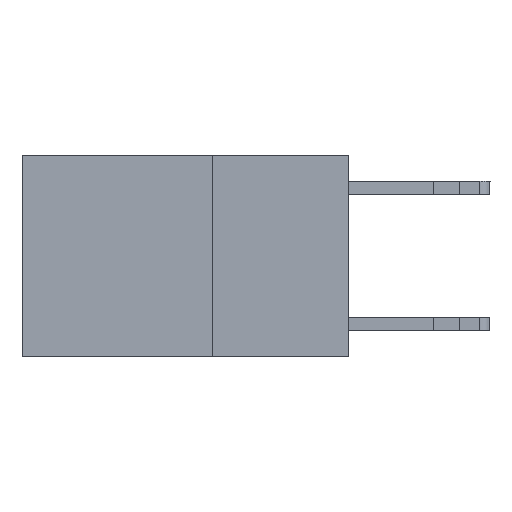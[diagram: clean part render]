
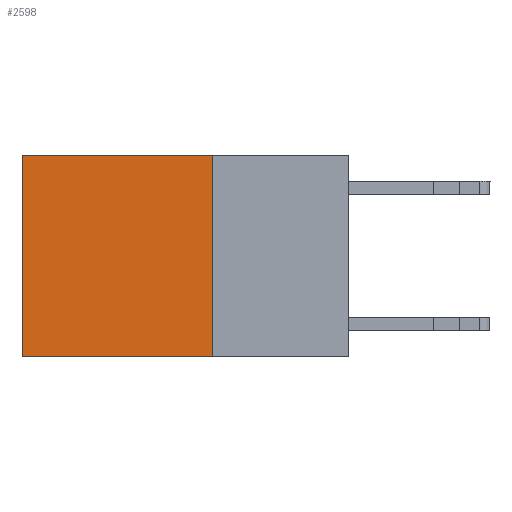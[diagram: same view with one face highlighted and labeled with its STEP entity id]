
A CAD part, left-side view. The second image highlights one B-rep face of the part: STEP entity #2598.
In plain terms, the highlighted planar face has unit normal (-1, 0, 0).
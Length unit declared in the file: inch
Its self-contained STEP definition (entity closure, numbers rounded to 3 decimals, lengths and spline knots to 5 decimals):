
#305 = EDGE_CURVE ( 'NONE', #5420, #4736, #16088, .T. ) ;
#388 = CARTESIAN_POINT ( 'NONE',  ( 0.2625, 0.25, -0.37 ) ) ;
#430 = EDGE_CURVE ( 'NONE', #694, #5420, #10399, .T. ) ;
#692 = ORIENTED_EDGE ( 'NONE', *, *, #13456, .F. ) ;
#694 = VERTEX_POINT ( 'NONE', #13172 ) ;
#736 = VECTOR ( 'NONE', #8948, 39.37008 ) ;
#1583 = DIRECTION ( 'NONE',  ( 0., 0., -1. ) ) ;
#2467 = ORIENTED_EDGE ( 'NONE', *, *, #305, .T. ) ;
#2598 = ADVANCED_FACE ( 'NONE', ( #13150 ), #17748, .F. ) ;
#3112 = CARTESIAN_POINT ( 'NONE',  ( 0.2625, 0.25, 0. ) ) ;
#3293 = DIRECTION ( 'NONE',  ( 0., 1., 0. ) ) ;
#4736 = VERTEX_POINT ( 'NONE', #14880 ) ;
#4841 = LINE ( 'NONE', #388, #7331 ) ;
#5153 = EDGE_LOOP ( 'NONE', ( #2467, #5311, #692, #10126 ) ) ;
#5311 = ORIENTED_EDGE ( 'NONE', *, *, #13603, .F. ) ;
#5420 = VERTEX_POINT ( 'NONE', #16393 ) ;
#5458 = DIRECTION ( 'NONE',  ( 0., 0., -1. ) ) ;
#6004 = CARTESIAN_POINT ( 'NONE',  ( 0.2625, 0.25, -0.37 ) ) ;
#6324 = VERTEX_POINT ( 'NONE', #6004 ) ;
#7014 = CARTESIAN_POINT ( 'NONE',  ( 0.2625, 0.6, 0. ) ) ;
#7331 = VECTOR ( 'NONE', #3293, 39.37008 ) ;
#7502 = DIRECTION ( 'NONE',  ( 0., 0., -1. ) ) ;
#8683 = CARTESIAN_POINT ( 'NONE',  ( 0.2625, 0.25, 0. ) ) ;
#8764 = LINE ( 'NONE', #16195, #13220 ) ;
#8948 = DIRECTION ( 'NONE',  ( 0., 1., 0. ) ) ;
#9087 = VECTOR ( 'NONE', #5458, 39.37008 ) ;
#10126 = ORIENTED_EDGE ( 'NONE', *, *, #430, .T. ) ;
#10399 = LINE ( 'NONE', #3112, #736 ) ;
#13150 = FACE_OUTER_BOUND ( 'NONE', #5153, .T. ) ;
#13172 = CARTESIAN_POINT ( 'NONE',  ( 0.2625, 0.25, 0. ) ) ;
#13220 = VECTOR ( 'NONE', #7502, 39.37008 ) ;
#13456 = EDGE_CURVE ( 'NONE', #694, #6324, #8764, .T. ) ;
#13603 = EDGE_CURVE ( 'NONE', #6324, #4736, #4841, .T. ) ;
#14731 = DIRECTION ( 'NONE',  ( 1., 0., 0. ) ) ;
#14880 = CARTESIAN_POINT ( 'NONE',  ( 0.2625, 0.6, -0.37 ) ) ;
#16088 = LINE ( 'NONE', #7014, #9087 ) ;
#16150 = AXIS2_PLACEMENT_3D ( 'NONE', #8683, #14731, #1583 ) ;
#16195 = CARTESIAN_POINT ( 'NONE',  ( 0.2625, 0.25, 0. ) ) ;
#16393 = CARTESIAN_POINT ( 'NONE',  ( 0.2625, 0.6, 0. ) ) ;
#17748 = PLANE ( 'NONE',  #16150 ) ;
